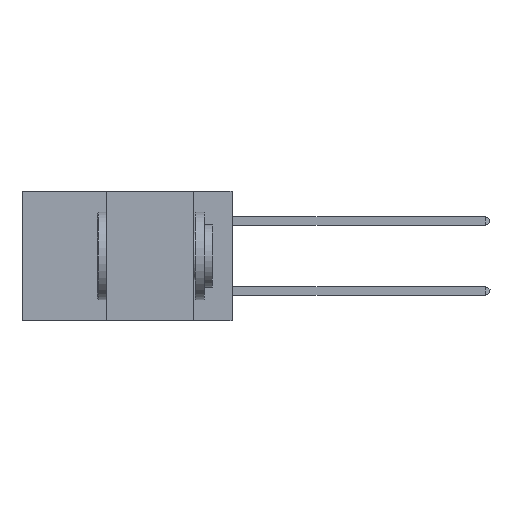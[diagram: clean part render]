
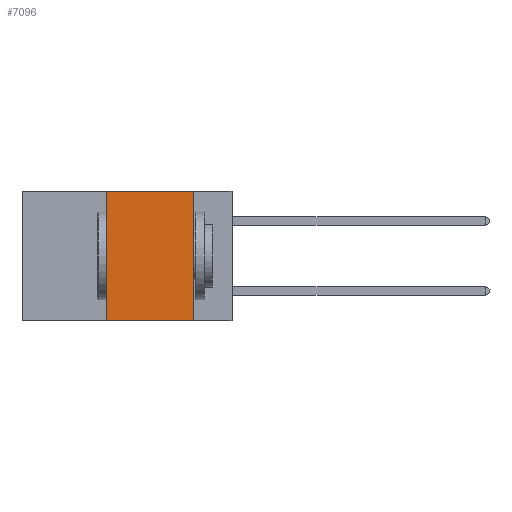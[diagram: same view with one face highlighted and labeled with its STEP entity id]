
A CAD part, left-side view. The second image highlights one B-rep face of the part: STEP entity #7096.
In plain terms, the highlighted planar face has unit normal (-1, 0, 0).
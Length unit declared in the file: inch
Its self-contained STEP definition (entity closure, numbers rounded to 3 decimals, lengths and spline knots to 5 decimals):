
#123 = VERTEX_POINT ( 'NONE', #3396 ) ;
#148 = CARTESIAN_POINT ( 'NONE',  ( 0., 0.6, 0. ) ) ;
#489 = DIRECTION ( 'NONE',  ( 0., 0., 1. ) ) ;
#1109 = CARTESIAN_POINT ( 'NONE',  ( 0., 0.6, -0.37 ) ) ;
#1536 = EDGE_CURVE ( 'NONE', #2104, #9844, #4685, .T. ) ;
#1936 = LINE ( 'NONE', #4159, #2717 ) ;
#1974 = DIRECTION ( 'NONE',  ( 0., 0., -1. ) ) ;
#2104 = VERTEX_POINT ( 'NONE', #4595 ) ;
#2542 = VECTOR ( 'NONE', #6962, 39.37008 ) ;
#2717 = VECTOR ( 'NONE', #1974, 39.37008 ) ;
#2760 = ORIENTED_EDGE ( 'NONE', *, *, #5780, .F. ) ;
#2781 = ORIENTED_EDGE ( 'NONE', *, *, #1536, .F. ) ;
#2957 = CARTESIAN_POINT ( 'NONE',  ( 0., 0.6, 0. ) ) ;
#3167 = AXIS2_PLACEMENT_3D ( 'NONE', #148, #3406, #7426 ) ;
#3396 = CARTESIAN_POINT ( 'NONE',  ( 0., 0.36, -0.37 ) ) ;
#3406 = DIRECTION ( 'NONE',  ( 1., 0., 0. ) ) ;
#4159 = CARTESIAN_POINT ( 'NONE',  ( 0., 0.11, 0. ) ) ;
#4423 = CARTESIAN_POINT ( 'NONE',  ( 0., 0.11, 0. ) ) ;
#4541 = EDGE_CURVE ( 'NONE', #123, #8012, #7210, .T. ) ;
#4595 = CARTESIAN_POINT ( 'NONE',  ( 0., 0.36, 0. ) ) ;
#4685 = LINE ( 'NONE', #2957, #2542 ) ;
#5233 = EDGE_LOOP ( 'NONE', ( #2760, #2781, #7762, #9327 ) ) ;
#5763 = CARTESIAN_POINT ( 'NONE',  ( 0., 0.11, -0.37 ) ) ;
#5780 = EDGE_CURVE ( 'NONE', #9844, #8012, #1936, .T. ) ;
#5881 = FACE_OUTER_BOUND ( 'NONE', #5233, .T. ) ;
#6689 = DIRECTION ( 'NONE',  ( 0., -1., 0. ) ) ;
#6736 = EDGE_CURVE ( 'NONE', #123, #2104, #9536, .T. ) ;
#6962 = DIRECTION ( 'NONE',  ( 0., -1., 0. ) ) ;
#7096 = ADVANCED_FACE ( 'NONE', ( #5881 ), #8198, .F. ) ;
#7210 = LINE ( 'NONE', #1109, #10134 ) ;
#7426 = DIRECTION ( 'NONE',  ( 0., 0., -1. ) ) ;
#7488 = VECTOR ( 'NONE', #489, 39.37008 ) ;
#7708 = CARTESIAN_POINT ( 'NONE',  ( 0., 0.36, 0. ) ) ;
#7762 = ORIENTED_EDGE ( 'NONE', *, *, #6736, .F. ) ;
#8012 = VERTEX_POINT ( 'NONE', #5763 ) ;
#8198 = PLANE ( 'NONE',  #3167 ) ;
#9327 = ORIENTED_EDGE ( 'NONE', *, *, #4541, .T. ) ;
#9536 = LINE ( 'NONE', #7708, #7488 ) ;
#9844 = VERTEX_POINT ( 'NONE', #4423 ) ;
#10134 = VECTOR ( 'NONE', #6689, 39.37008 ) ;
